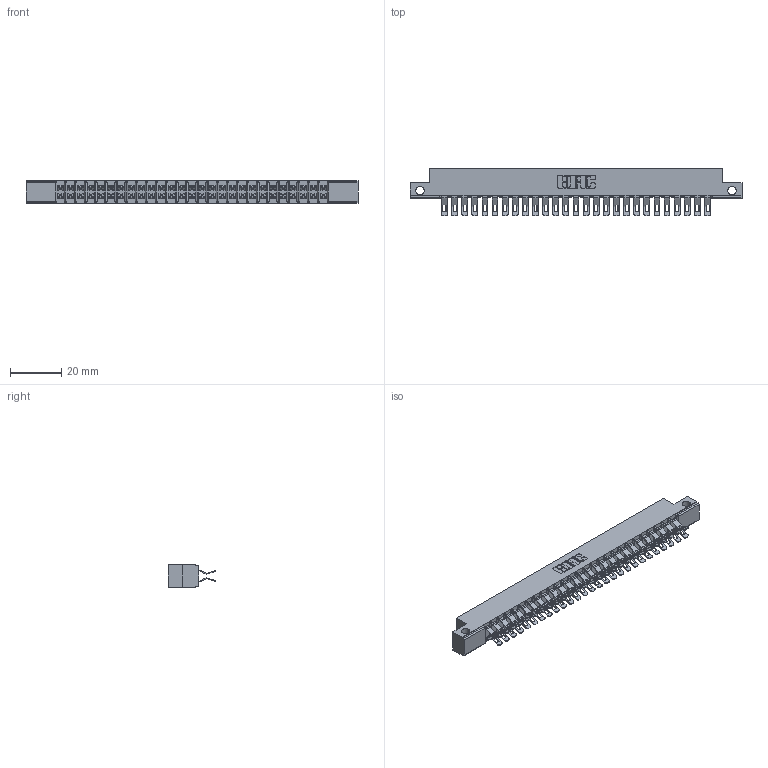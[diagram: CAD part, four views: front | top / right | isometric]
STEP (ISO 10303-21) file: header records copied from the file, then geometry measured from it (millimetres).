
FILE_DESCRIPTION (( 'STEP AP203' ), '1' );
FILE_NAME ('357-054-455-212.STEP', '2020-10-04T08:57:46', ( '' ), ( '' ), 'SwSTEP 2.0', 'SolidWorks 2020', '' );
FILE_SCHEMA (( 'CONFIG_CONTROL_DESIGN' ));
Length unit declared in the file: inch
Products named in the file (3): 357-054-455-212; 307 Part_.128 Dia Side Mounting Holes; 307-290-001_555
Assembly tree (55 placements, depth 2):
  357-054-455-212
    307 Part_.128 Dia Side Mounting Holes
    307-290-001_555  x54
Bounding box: 130 x 18.75 x 8.71 mm (x, y, z)
Volume: 8587.6 mm3; surface area: 16178.9 mm2
Topology: 55 solids, 55 shells, 3440 faces, 10097 edges, 6582 vertices
Faces by surface type: plane 1906, cylinder 1478, sphere 56
Entity records: 26399 total; most frequent: CARTESIAN_POINT 4327, ORIENTED_EDGE 4288, DIRECTION 4252, EDGE_CURVE 2144, VECTOR 1626, LINE 1626, VERTEX_POINT 1388, AXIS2_PLACEMENT_3D 1313
